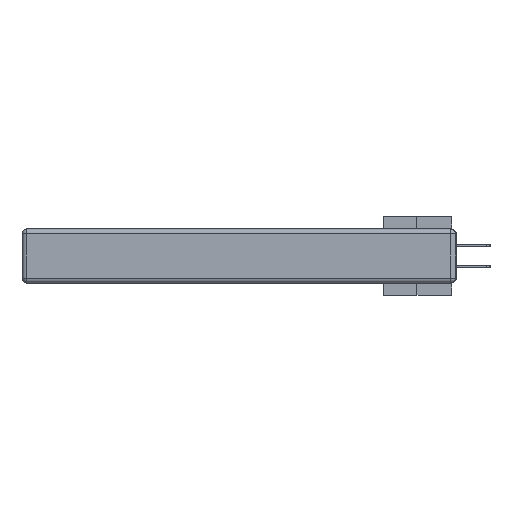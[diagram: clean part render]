
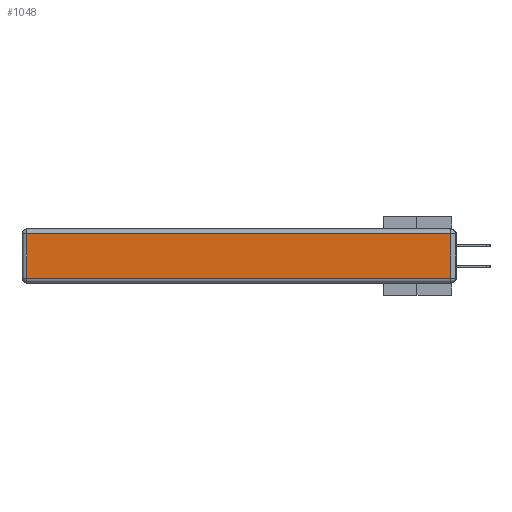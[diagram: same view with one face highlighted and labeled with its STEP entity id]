
A CAD part, left-side view. The second image highlights one B-rep face of the part: STEP entity #1048.
In plain terms, the highlighted planar face has unit normal (-1, 0, 0).
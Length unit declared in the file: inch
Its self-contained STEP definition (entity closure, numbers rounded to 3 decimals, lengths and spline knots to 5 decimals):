
#304 = CARTESIAN_POINT ( 'NONE',  ( 0., 2.72, -0.343 ) ) ;
#528 = ORIENTED_EDGE ( 'NONE', *, *, #1589, .T. ) ;
#1048 = ADVANCED_FACE ( 'NONE', ( #19261 ), #16782, .T. ) ;
#1246 = DIRECTION ( 'NONE',  ( -1., 0., 0. ) ) ;
#1411 = VECTOR ( 'NONE', #31093, 39.37008 ) ;
#1589 = EDGE_CURVE ( 'NONE', #34213, #23386, #24207, .T. ) ;
#3636 = ORIENTED_EDGE ( 'NONE', *, *, #12101, .T. ) ;
#4075 = CARTESIAN_POINT ( 'NONE',  ( 0., 2.75, -0.03 ) ) ;
#4471 = CARTESIAN_POINT ( 'NONE',  ( 0., 0., -0.313 ) ) ;
#4527 = ORIENTED_EDGE ( 'NONE', *, *, #11859, .T. ) ;
#4857 = LINE ( 'NONE', #4471, #33290 ) ;
#7489 = CARTESIAN_POINT ( 'NONE',  ( 0., 0.03, -0.343 ) ) ;
#9492 = DIRECTION ( 'NONE',  ( 0., 1., 0. ) ) ;
#10731 = VERTEX_POINT ( 'NONE', #16261 ) ;
#11859 = EDGE_CURVE ( 'NONE', #20034, #34213, #25295, .T. ) ;
#12101 = EDGE_CURVE ( 'NONE', #23386, #10731, #29903, .T. ) ;
#14011 = VECTOR ( 'NONE', #27337, 39.37008 ) ;
#16261 = CARTESIAN_POINT ( 'NONE',  ( 0., 2.72, -0.313 ) ) ;
#16551 = EDGE_LOOP ( 'NONE', ( #31151, #4527, #528, #3636 ) ) ;
#16782 = PLANE ( 'NONE',  #29517 ) ;
#19182 = CARTESIAN_POINT ( 'NONE',  ( 0., 2.72, -0.03 ) ) ;
#19261 = FACE_OUTER_BOUND ( 'NONE', #16551, .T. ) ;
#20034 = VERTEX_POINT ( 'NONE', #25854 ) ;
#20444 = VECTOR ( 'NONE', #9492, 39.37008 ) ;
#22328 = DIRECTION ( 'NONE',  ( 0., 0., 1. ) ) ;
#22865 = EDGE_CURVE ( 'NONE', #10731, #20034, #4857, .T. ) ;
#23386 = VERTEX_POINT ( 'NONE', #19182 ) ;
#24207 = LINE ( 'NONE', #4075, #20444 ) ;
#24572 = CARTESIAN_POINT ( 'NONE',  ( 0., 0.03, -0.03 ) ) ;
#25295 = LINE ( 'NONE', #7489, #1411 ) ;
#25854 = CARTESIAN_POINT ( 'NONE',  ( 0., 0.03, -0.313 ) ) ;
#27337 = DIRECTION ( 'NONE',  ( 0., 0., -1. ) ) ;
#29517 = AXIS2_PLACEMENT_3D ( 'NONE', #30653, #1246, #22328 ) ;
#29903 = LINE ( 'NONE', #304, #14011 ) ;
#30653 = CARTESIAN_POINT ( 'NONE',  ( 0., 0., -0.343 ) ) ;
#30679 = DIRECTION ( 'NONE',  ( 0., -1., 0. ) ) ;
#31093 = DIRECTION ( 'NONE',  ( 0., 0., 1. ) ) ;
#31151 = ORIENTED_EDGE ( 'NONE', *, *, #22865, .T. ) ;
#33290 = VECTOR ( 'NONE', #30679, 39.37008 ) ;
#34213 = VERTEX_POINT ( 'NONE', #24572 ) ;
